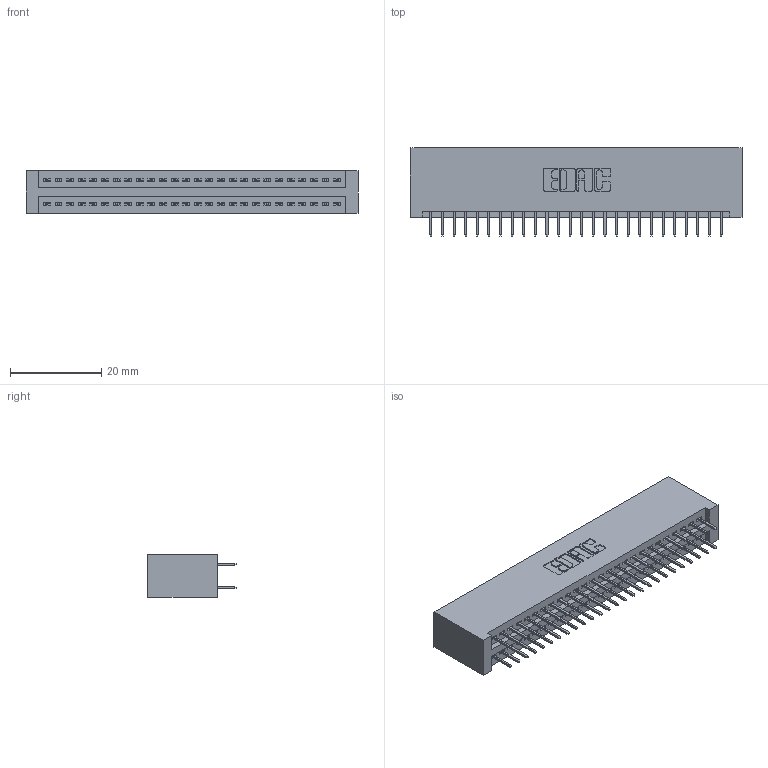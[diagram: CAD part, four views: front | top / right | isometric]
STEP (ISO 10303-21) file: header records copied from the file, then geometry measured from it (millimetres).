
FILE_DESCRIPTION (( 'STEP AP203' ), '1' );
FILE_NAME ('395-052-524-201.STEP', '2018-11-20T22:29:03', ( '' ), ( '' ), 'SwSTEP 2.0', 'SolidWorks 2016', '' );
FILE_SCHEMA (( 'CONFIG_CONTROL_DESIGN' ));
Length unit declared in the file: inch
Products named in the file (3): 345-292-001_345-293-124; 345 Part_No Mounting Lugs; 395-052-524-201
Assembly tree (53 placements, depth 2):
  395-052-524-201
    345 Part_No Mounting Lugs
    345-292-001_345-293-124  x52
Bounding box: 72.64 x 19.35 x 9.4 mm (x, y, z)
Volume: 7445.4 mm3; surface area: 10791.2 mm2
Topology: 53 solids, 53 shells, 2926 faces, 8273 edges, 5306 vertices
Faces by surface type: plane 2104, cylinder 822
Entity records: 22351 total; most frequent: CARTESIAN_POINT 3760, ORIENTED_EDGE 3694, DIRECTION 3331, EDGE_CURVE 1847, VECTOR 1623, LINE 1623, VERTEX_POINT 1226, AXIS2_PLACEMENT_3D 854
